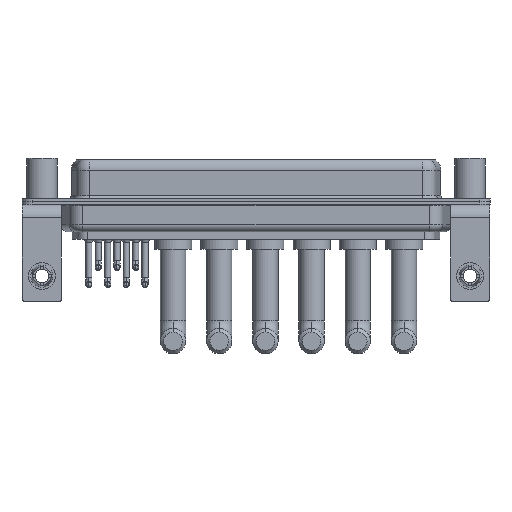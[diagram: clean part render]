
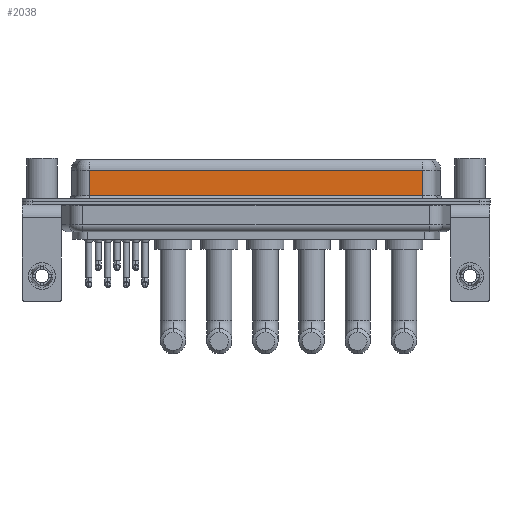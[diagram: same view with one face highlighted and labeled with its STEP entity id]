
A CAD part, front view. The second image highlights one B-rep face of the part: STEP entity #2038.
In plain terms, the highlighted planar face has unit normal (0, -1, 0).
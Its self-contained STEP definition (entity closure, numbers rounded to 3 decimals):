
#1605 = CARTESIAN_POINT ( 'NONE',  ( 56.462, -3.95, 4.65 ) ) ;
#1660 = DIRECTION ( 'NONE',  ( 0., 0., 1. ) ) ;
#2038 = ADVANCED_FACE ( 'NONE', ( #3161 ), #5302, .F. ) ;
#2726 = CARTESIAN_POINT ( 'NONE',  ( 56.462, -3.95, 0.9 ) ) ;
#2858 = DIRECTION ( 'NONE',  ( 0., 0., -1. ) ) ;
#3161 = FACE_OUTER_BOUND ( 'NONE', #15110, .T. ) ;
#4415 = DIRECTION ( 'NONE',  ( 1., 0., 0. ) ) ;
#4658 = LINE ( 'NONE', #13218, #22212 ) ;
#4678 = EDGE_CURVE ( 'NONE', #14429, #21173, #6151, .T. ) ;
#5302 = PLANE ( 'NONE',  #16250 ) ;
#5332 = VECTOR ( 'NONE', #16812, 1000. ) ;
#5619 = VECTOR ( 'NONE', #19694, 1000. ) ;
#5812 = CARTESIAN_POINT ( 'NONE',  ( 56.462, -3.95, 4.65 ) ) ;
#5999 = ORIENTED_EDGE ( 'NONE', *, *, #11818, .T. ) ;
#6151 = LINE ( 'NONE', #2726, #8957 ) ;
#6260 = VERTEX_POINT ( 'NONE', #1605 ) ;
#6500 = CARTESIAN_POINT ( 'NONE',  ( 56.462, -3.95, 0.9 ) ) ;
#6807 = DIRECTION ( 'NONE',  ( 0., 1., 0. ) ) ;
#7257 = ORIENTED_EDGE ( 'NONE', *, *, #16021, .T. ) ;
#7458 = ORIENTED_EDGE ( 'NONE', *, *, #20986, .F. ) ;
#8102 = LINE ( 'NONE', #5812, #5619 ) ;
#8631 = CARTESIAN_POINT ( 'NONE',  ( 7.038, -3.95, 6.4 ) ) ;
#8868 = CARTESIAN_POINT ( 'NONE',  ( 7.038, -3.95, 0.9 ) ) ;
#8957 = VECTOR ( 'NONE', #4415, 1000. ) ;
#9716 = CARTESIAN_POINT ( 'NONE',  ( 7.038, -3.95, 4.65 ) ) ;
#9879 = LINE ( 'NONE', #8631, #5332 ) ;
#11818 = EDGE_CURVE ( 'NONE', #6260, #21940, #8102, .T. ) ;
#13218 = CARTESIAN_POINT ( 'NONE',  ( 56.462, -3.95, 6.4 ) ) ;
#13754 = CARTESIAN_POINT ( 'NONE',  ( 56.462, -3.95, 6.4 ) ) ;
#14429 = VERTEX_POINT ( 'NONE', #8868 ) ;
#15110 = EDGE_LOOP ( 'NONE', ( #7458, #5999, #7257, #19647 ) ) ;
#16021 = EDGE_CURVE ( 'NONE', #21940, #14429, #9879, .T. ) ;
#16250 = AXIS2_PLACEMENT_3D ( 'NONE', #13754, #6807, #1660 ) ;
#16812 = DIRECTION ( 'NONE',  ( 0., 0., -1. ) ) ;
#19647 = ORIENTED_EDGE ( 'NONE', *, *, #4678, .T. ) ;
#19694 = DIRECTION ( 'NONE',  ( -1., 0., 0. ) ) ;
#20986 = EDGE_CURVE ( 'NONE', #6260, #21173, #4658, .T. ) ;
#21173 = VERTEX_POINT ( 'NONE', #6500 ) ;
#21940 = VERTEX_POINT ( 'NONE', #9716 ) ;
#22212 = VECTOR ( 'NONE', #2858, 1000. ) ;
